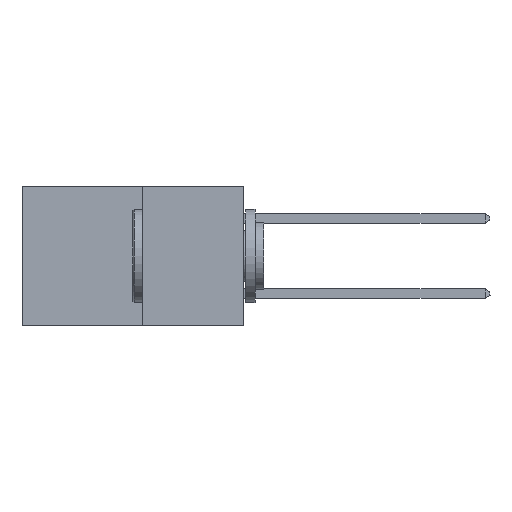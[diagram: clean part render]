
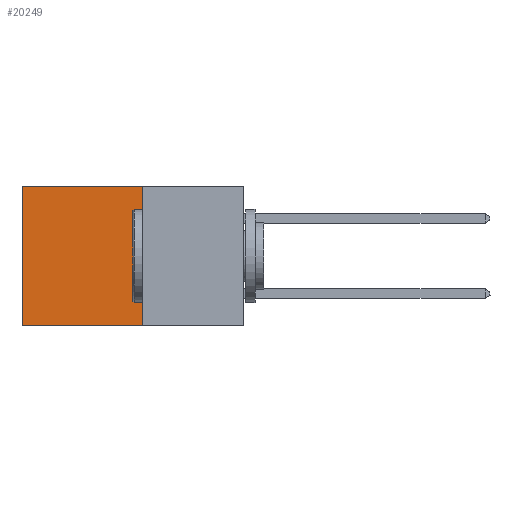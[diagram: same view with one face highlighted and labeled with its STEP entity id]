
A CAD part, left-side view. The second image highlights one B-rep face of the part: STEP entity #20249.
In plain terms, the highlighted planar face has unit normal (-1, 0, 0).
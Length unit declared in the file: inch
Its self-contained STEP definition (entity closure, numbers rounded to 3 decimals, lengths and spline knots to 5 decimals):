
#3467 = VERTEX_POINT ( 'NONE', #19136 ) ;
#4130 = CARTESIAN_POINT ( 'NONE',  ( 0.277, 0.27, -0.37 ) ) ;
#5634 = EDGE_CURVE ( 'NONE', #27724, #26500, #14544, .T. ) ;
#6104 = LINE ( 'NONE', #23884, #32150 ) ;
#9160 = AXIS2_PLACEMENT_3D ( 'NONE', #29605, #14620, #32112 ) ;
#9487 = VERTEX_POINT ( 'NONE', #29775 ) ;
#12936 = CARTESIAN_POINT ( 'NONE',  ( 0.277, 0.27, 0. ) ) ;
#12942 = DIRECTION ( 'NONE',  ( 0., 1., 0. ) ) ;
#13817 = EDGE_CURVE ( 'NONE', #27724, #9487, #23329, .T. ) ;
#13827 = DIRECTION ( 'NONE',  ( 0., 0., -1. ) ) ;
#14544 = LINE ( 'NONE', #12936, #27880 ) ;
#14620 = DIRECTION ( 'NONE',  ( 1., 0., 0. ) ) ;
#15225 = CARTESIAN_POINT ( 'NONE',  ( 0.277, 0.59, 0. ) ) ;
#18017 = EDGE_CURVE ( 'NONE', #26500, #3467, #6104, .T. ) ;
#18978 = EDGE_LOOP ( 'NONE', ( #19935, #23936, #27386, #22885 ) ) ;
#19136 = CARTESIAN_POINT ( 'NONE',  ( 0.277, 0.59, -0.37 ) ) ;
#19935 = ORIENTED_EDGE ( 'NONE', *, *, #18017, .T. ) ;
#20249 = ADVANCED_FACE ( 'NONE', ( #26601 ), #24638, .F. ) ;
#20768 = EDGE_CURVE ( 'NONE', #9487, #3467, #23115, .T. ) ;
#22710 = CARTESIAN_POINT ( 'NONE',  ( 0.277, 0.27, -0.37 ) ) ;
#22885 = ORIENTED_EDGE ( 'NONE', *, *, #5634, .T. ) ;
#23115 = LINE ( 'NONE', #22710, #31263 ) ;
#23318 = CARTESIAN_POINT ( 'NONE',  ( 0.277, 0.27, 0. ) ) ;
#23329 = LINE ( 'NONE', #4130, #29128 ) ;
#23884 = CARTESIAN_POINT ( 'NONE',  ( 0.277, 0.59, -0.37 ) ) ;
#23936 = ORIENTED_EDGE ( 'NONE', *, *, #20768, .F. ) ;
#24489 = DIRECTION ( 'NONE',  ( 0., 0., -1. ) ) ;
#24638 = PLANE ( 'NONE',  #9160 ) ;
#25221 = DIRECTION ( 'NONE',  ( 0., 1., 0. ) ) ;
#26500 = VERTEX_POINT ( 'NONE', #15225 ) ;
#26601 = FACE_OUTER_BOUND ( 'NONE', #18978, .T. ) ;
#27386 = ORIENTED_EDGE ( 'NONE', *, *, #13817, .F. ) ;
#27724 = VERTEX_POINT ( 'NONE', #23318 ) ;
#27880 = VECTOR ( 'NONE', #12942, 39.37008 ) ;
#29128 = VECTOR ( 'NONE', #24489, 39.37008 ) ;
#29605 = CARTESIAN_POINT ( 'NONE',  ( 0.277, 0.27, -0.37 ) ) ;
#29775 = CARTESIAN_POINT ( 'NONE',  ( 0.277, 0.27, -0.37 ) ) ;
#31263 = VECTOR ( 'NONE', #25221, 39.37008 ) ;
#32112 = DIRECTION ( 'NONE',  ( 0., 0., -1. ) ) ;
#32150 = VECTOR ( 'NONE', #13827, 39.37008 ) ;
